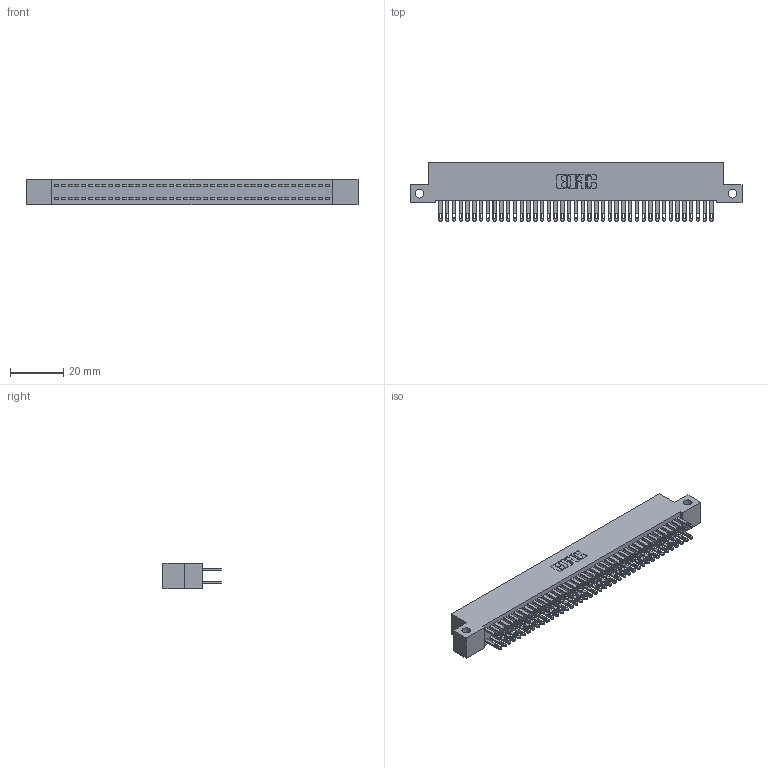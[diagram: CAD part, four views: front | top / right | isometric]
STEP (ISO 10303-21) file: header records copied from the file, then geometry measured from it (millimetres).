
FILE_DESCRIPTION (( 'STEP AP203' ), '1' );
FILE_NAME ('892-082-500-212.STEP', '2020-09-21T20:21:26', ( '' ), ( '' ), 'SwSTEP 2.0', 'SolidWorks 2020', '' );
FILE_SCHEMA (( 'CONFIG_CONTROL_DESIGN' ));
Length unit declared in the file: inch
Products named in the file (3): 842 Part_Side Mount; 892-082-500-212; 345-292-001_345-293-100
Assembly tree (83 placements, depth 2):
  892-082-500-212
    842 Part_Side Mount
    345-292-001_345-293-100  x82
Bounding box: 124.46 x 21.85 x 9.4 mm (x, y, z)
Volume: 11354.6 mm3; surface area: 19083.2 mm2
Topology: 83 solids, 83 shells, 4046 faces, 12353 edges, 8234 vertices
Faces by surface type: plane 2526, cylinder 1520
Entity records: 26307 total; most frequent: CARTESIAN_POINT 4358, ORIENTED_EDGE 4294, DIRECTION 3727, EDGE_CURVE 2147, VECTOR 2015, LINE 2015, VERTEX_POINT 1430, AXIS2_PLACEMENT_3D 856
